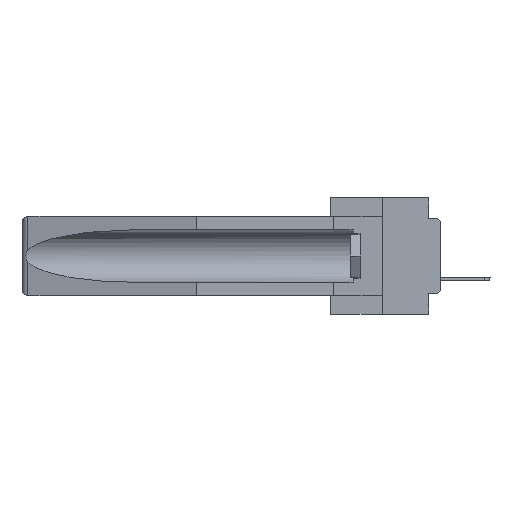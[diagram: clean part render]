
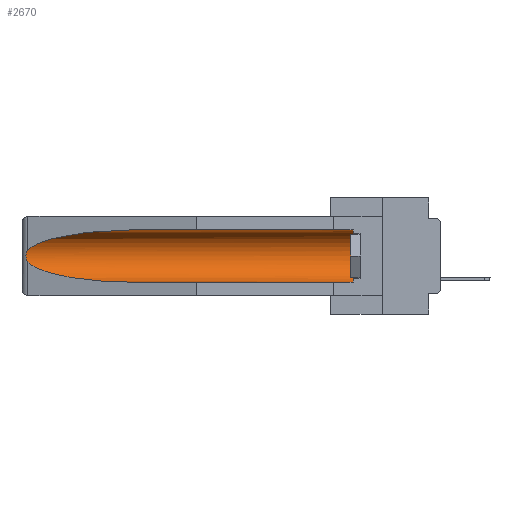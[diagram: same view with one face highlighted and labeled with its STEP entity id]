
A CAD part, left-side view. The second image highlights one B-rep face of the part: STEP entity #2670.
In plain terms, the highlighted cylindrical face has radius 2.857 mm (diameter 5.715 mm), a partial arc.
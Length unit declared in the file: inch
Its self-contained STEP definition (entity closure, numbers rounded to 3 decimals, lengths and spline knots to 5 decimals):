
#248 = AXIS2_PLACEMENT_3D ( 'NONE', #20349, #24438, #18274 ) ;
#349 = CARTESIAN_POINT ( 'NONE',  ( 0.155, 0.126, -0.059 ) ) ;
#1211 = ORIENTED_EDGE ( 'NONE', *, *, #11941, .T. ) ;
#1844 = CARTESIAN_POINT ( 'NONE',  ( 0.155, 1.07973, -0.059 ) ) ;
#1969 = CARTESIAN_POINT ( 'NONE',  ( 0.155, 1.07973, -0.284 ) ) ;
#2107 =( BOUNDED_CURVE ( )  B_SPLINE_CURVE ( 3, ( #9149, #17562, #15733, #4897 ),
 .UNSPECIFIED., .F., .F. ) 
 B_SPLINE_CURVE_WITH_KNOTS ( ( 4, 4 ),
 ( 0.1948, 1.5708 ),
 .UNSPECIFIED. ) 
 CURVE ( )  GEOMETRIC_REPRESENTATION_ITEM ( )  RATIONAL_B_SPLINE_CURVE ( ( 1., 0.848, 0.848, 1. ) ) 
 REPRESENTATION_ITEM ( '' )  );
#2138 = CARTESIAN_POINT ( 'NONE',  ( 0.25451, 1.48313, -0.09465 ) ) ;
#2670 = ADVANCED_FACE ( 'NONE', ( #27998 ), #6893, .F. ) ;
#3190 = DIRECTION ( 'NONE',  ( 0., -1., 0. ) ) ;
#4300 = CARTESIAN_POINT ( 'NONE',  ( 0.26537, 1.52718, -0.14972 ) ) ;
#4681 = CARTESIAN_POINT ( 'NONE',  ( 0.2675, 1.53308, -0.17534 ) ) ;
#4897 = CARTESIAN_POINT ( 'NONE',  ( 0.155, 1.07973, -0.284 ) ) ;
#5071 = LINE ( 'NONE', #24138, #10151 ) ;
#5435 = EDGE_CURVE ( 'NONE', #15408, #10162, #19706, .T. ) ;
#6199 = VERTEX_POINT ( 'NONE', #20014 ) ;
#6460 = CARTESIAN_POINT ( 'NONE',  ( 0.26537, 1.52718, -0.14972 ) ) ;
#6893 = CYLINDRICAL_SURFACE ( 'NONE', #248, 0.1125 ) ;
#7430 = CARTESIAN_POINT ( 'NONE',  ( 0.155, 0.126, -0.284 ) ) ;
#8306 = ORIENTED_EDGE ( 'NONE', *, *, #11994, .F. ) ;
#8863 = CARTESIAN_POINT ( 'NONE',  ( 0.26537, 1.52718, -0.19328 ) ) ;
#9149 = CARTESIAN_POINT ( 'NONE',  ( 0.26537, 1.52718, -0.19328 ) ) ;
#10151 = VECTOR ( 'NONE', #23962, 39.37008 ) ;
#10162 = VERTEX_POINT ( 'NONE', #12195 ) ;
#10853 = CARTESIAN_POINT ( 'NONE',  ( 0.26597, 1.52961, -0.15275 ) ) ;
#10945 = CARTESIAN_POINT ( 'NONE',  ( 0.26654, 1.53092, -0.15636 ) ) ;
#11275 = ORIENTED_EDGE ( 'NONE', *, *, #16599, .T. ) ;
#11941 = EDGE_CURVE ( 'NONE', #6199, #17075, #24866, .T. ) ;
#11994 = EDGE_CURVE ( 'NONE', #19918, #21923, #5071, .T. ) ;
#12195 = CARTESIAN_POINT ( 'NONE',  ( 0.155, 1.07973, -0.059 ) ) ;
#12198 = ORIENTED_EDGE ( 'NONE', *, *, #5435, .T. ) ;
#13138 = EDGE_CURVE ( 'NONE', #17075, #21923, #2107, .T. ) ;
#14071 = ORIENTED_EDGE ( 'NONE', *, *, #13138, .T. ) ;
#14185 = CARTESIAN_POINT ( 'NONE',  ( 0.155, 0.126, -0.1715 ) ) ;
#15408 = VERTEX_POINT ( 'NONE', #349 ) ;
#15733 = CARTESIAN_POINT ( 'NONE',  ( 0.21114, 1.30732, -0.284 ) ) ;
#15782 = EDGE_CURVE ( 'NONE', #10162, #6199, #20178, .T. ) ;
#16092 = DIRECTION ( 'NONE',  ( 0., 0., 1. ) ) ;
#16599 = EDGE_CURVE ( 'NONE', #19918, #15408, #22194, .T. ) ;
#17075 = VERTEX_POINT ( 'NONE', #8863 ) ;
#17523 = CARTESIAN_POINT ( 'NONE',  ( 0.2673, 1.5327, -0.16383 ) ) ;
#17562 = CARTESIAN_POINT ( 'NONE',  ( 0.25451, 1.48313, -0.24835 ) ) ;
#18274 = DIRECTION ( 'NONE',  ( 0., 0., 1. ) ) ;
#19118 = CARTESIAN_POINT ( 'NONE',  ( 0.21114, 1.30732, -0.059 ) ) ;
#19287 = EDGE_LOOP ( 'NONE', ( #25093, #1211, #14071, #8306, #11275, #12198 ) ) ;
#19588 = CARTESIAN_POINT ( 'NONE',  ( 0.2673, 1.53269, -0.17917 ) ) ;
#19706 = LINE ( 'NONE', #23402, #20023 ) ;
#19918 = VERTEX_POINT ( 'NONE', #7430 ) ;
#20014 = CARTESIAN_POINT ( 'NONE',  ( 0.26537, 1.52718, -0.14972 ) ) ;
#20023 = VECTOR ( 'NONE', #23784, 39.37008 ) ;
#20178 =( BOUNDED_CURVE ( )  B_SPLINE_CURVE ( 3, ( #1844, #19118, #2138, #4300 ),
 .UNSPECIFIED., .F., .F. ) 
 B_SPLINE_CURVE_WITH_KNOTS ( ( 4, 4 ),
 ( 4.71239, 6.08839 ),
 .UNSPECIFIED. ) 
 CURVE ( )  GEOMETRIC_REPRESENTATION_ITEM ( )  RATIONAL_B_SPLINE_CURVE ( ( 1., 0.848, 0.848, 1. ) ) 
 REPRESENTATION_ITEM ( '' )  );
#20349 = CARTESIAN_POINT ( 'NONE',  ( 0.155, -0.30754, -0.1715 ) ) ;
#21774 = CARTESIAN_POINT ( 'NONE',  ( 0.26655, 1.53094, -0.18657 ) ) ;
#21923 = VERTEX_POINT ( 'NONE', #1969 ) ;
#22194 = CIRCLE ( 'NONE', #27798, 0.1125 ) ;
#23402 = CARTESIAN_POINT ( 'NONE',  ( 0.155, -0.30754, -0.059 ) ) ;
#23784 = DIRECTION ( 'NONE',  ( 0., 1., 0. ) ) ;
#23868 = CARTESIAN_POINT ( 'NONE',  ( 0.26597, 1.5296, -0.19026 ) ) ;
#23962 = DIRECTION ( 'NONE',  ( 0., 1., 0. ) ) ;
#24138 = CARTESIAN_POINT ( 'NONE',  ( 0.155, -0.30754, -0.284 ) ) ;
#24233 = CARTESIAN_POINT ( 'NONE',  ( 0.26537, 1.52718, -0.19328 ) ) ;
#24438 = DIRECTION ( 'NONE',  ( 0., 1., 0. ) ) ;
#24866 = B_SPLINE_CURVE_WITH_KNOTS ( 'NONE', 3,
 ( #6460, #10853, #10945, #17523, #26421, #4681, #19588, #21774, #23868, #24233 ),
 .UNSPECIFIED., .F., .F.,
 ( 4, 2, 2, 2, 4 ),
 ( 0., 0.00029, 0.00058, 0.00087, 0.00117 ),
 .UNSPECIFIED. ) ;
#25093 = ORIENTED_EDGE ( 'NONE', *, *, #15782, .T. ) ;
#26421 = CARTESIAN_POINT ( 'NONE',  ( 0.2675, 1.53308, -0.16763 ) ) ;
#27798 = AXIS2_PLACEMENT_3D ( 'NONE', #14185, #3190, #16092 ) ;
#27998 = FACE_OUTER_BOUND ( 'NONE', #19287, .T. ) ;
